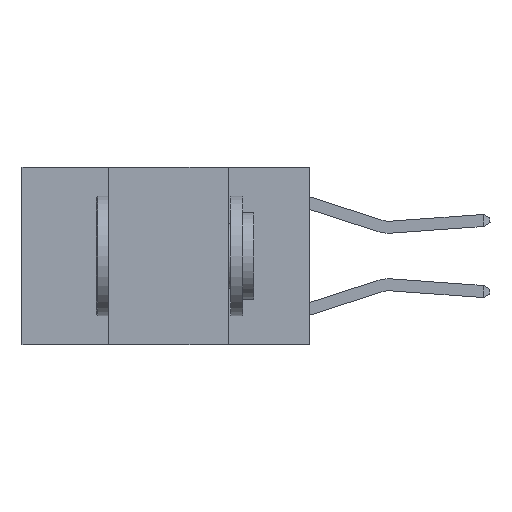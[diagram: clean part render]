
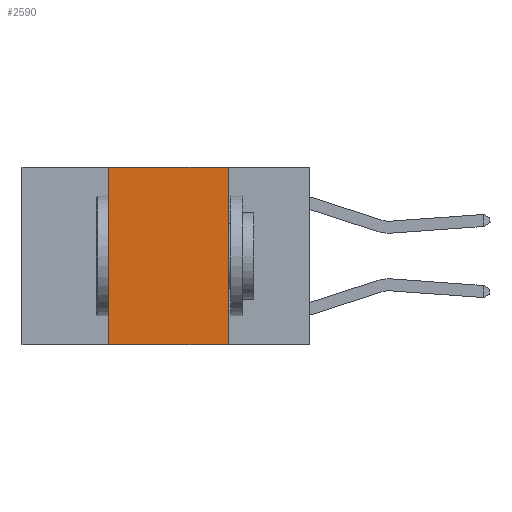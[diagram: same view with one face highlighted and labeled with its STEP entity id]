
A CAD part, left-side view. The second image highlights one B-rep face of the part: STEP entity #2590.
In plain terms, the highlighted planar face has unit normal (-1, 0, 0).
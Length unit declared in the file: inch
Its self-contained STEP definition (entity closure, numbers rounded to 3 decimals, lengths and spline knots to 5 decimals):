
#63 = VECTOR ( 'NONE', #291, 39.37008 ) ;
#74 = VERTEX_POINT ( 'NONE', #8875 ) ;
#291 = DIRECTION ( 'NONE',  ( 0., -1., 0. ) ) ;
#440 = VECTOR ( 'NONE', #7502, 39.37008 ) ;
#1069 = ORIENTED_EDGE ( 'NONE', *, *, #2470, .F. ) ;
#1084 = ORIENTED_EDGE ( 'NONE', *, *, #4734, .F. ) ;
#1393 = ORIENTED_EDGE ( 'NONE', *, *, #9462, .T. ) ;
#1592 = DIRECTION ( 'NONE',  ( 0., 0., -1. ) ) ;
#1600 = FACE_OUTER_BOUND ( 'NONE', #10564, .T. ) ;
#1694 = DIRECTION ( 'NONE',  ( 0., -1., 0. ) ) ;
#1887 = CARTESIAN_POINT ( 'NONE',  ( 0., 0.17, -0.37 ) ) ;
#2188 = LINE ( 'NONE', #8959, #9192 ) ;
#2236 = ORIENTED_EDGE ( 'NONE', *, *, #3532, .F. ) ;
#2457 = LINE ( 'NONE', #11611, #9155 ) ;
#2470 = EDGE_CURVE ( 'NONE', #4392, #74, #5710, .T. ) ;
#2590 = ADVANCED_FACE ( 'NONE', ( #1600 ), #4072, .F. ) ;
#3258 = AXIS2_PLACEMENT_3D ( 'NONE', #3917, #3803, #3735 ) ;
#3532 = EDGE_CURVE ( 'NONE', #11764, #6429, #2188, .T. ) ;
#3735 = DIRECTION ( 'NONE',  ( 0., 0., -1. ) ) ;
#3803 = DIRECTION ( 'NONE',  ( 1., 0., 0. ) ) ;
#3917 = CARTESIAN_POINT ( 'NONE',  ( 0., 0.6, 0. ) ) ;
#4072 = PLANE ( 'NONE',  #3258 ) ;
#4392 = VERTEX_POINT ( 'NONE', #6914 ) ;
#4734 = EDGE_CURVE ( 'NONE', #74, #11764, #2457, .T. ) ;
#5710 = LINE ( 'NONE', #8168, #440 ) ;
#6429 = VERTEX_POINT ( 'NONE', #1887 ) ;
#6914 = CARTESIAN_POINT ( 'NONE',  ( 0., 0.42, -0.37 ) ) ;
#7055 = CARTESIAN_POINT ( 'NONE',  ( 0., 0.6, -0.37 ) ) ;
#7502 = DIRECTION ( 'NONE',  ( 0., 0., 1. ) ) ;
#7837 = CARTESIAN_POINT ( 'NONE',  ( 0., 0.17, 0. ) ) ;
#8168 = CARTESIAN_POINT ( 'NONE',  ( 0., 0.42, 0. ) ) ;
#8875 = CARTESIAN_POINT ( 'NONE',  ( 0., 0.42, 0. ) ) ;
#8959 = CARTESIAN_POINT ( 'NONE',  ( 0., 0.17, 0. ) ) ;
#9155 = VECTOR ( 'NONE', #1694, 39.37008 ) ;
#9192 = VECTOR ( 'NONE', #1592, 39.37008 ) ;
#9462 = EDGE_CURVE ( 'NONE', #4392, #6429, #10309, .T. ) ;
#10309 = LINE ( 'NONE', #7055, #63 ) ;
#10564 = EDGE_LOOP ( 'NONE', ( #2236, #1084, #1069, #1393 ) ) ;
#11611 = CARTESIAN_POINT ( 'NONE',  ( 0., 0.6, 0. ) ) ;
#11764 = VERTEX_POINT ( 'NONE', #7837 ) ;
